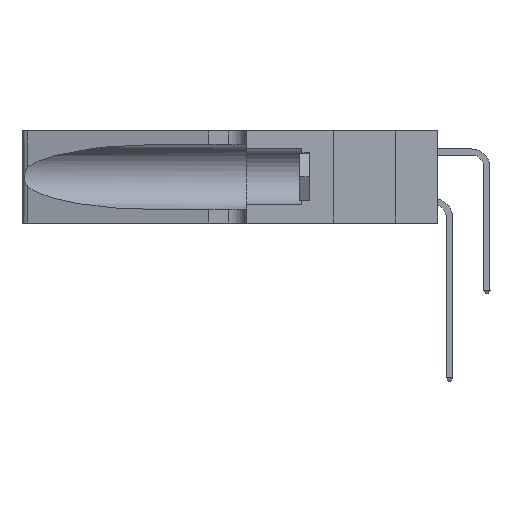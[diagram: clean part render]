
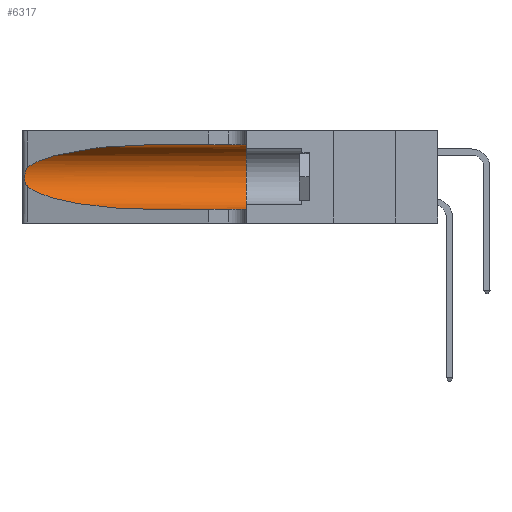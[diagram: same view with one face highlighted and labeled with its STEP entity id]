
A CAD part, left-side view. The second image highlights one B-rep face of the part: STEP entity #6317.
In plain terms, the highlighted cylindrical face has radius 3.308 mm (diameter 6.617 mm), a partial arc.
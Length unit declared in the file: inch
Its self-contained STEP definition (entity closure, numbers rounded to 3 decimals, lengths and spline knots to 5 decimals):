
#1253 = B_SPLINE_CURVE_WITH_KNOTS ( 'NONE', 3,
 ( #28979, #22454, #2146, #24443, #17935, #11226, #15744, #15454, #1946, #20018, #22271, #10839, #24629, #8746 ),
 .UNSPECIFIED., .F., .F.,
 ( 4, 2, 2, 2, 2, 2, 4 ),
 ( 0., 0.00027, 0.00053, 0.00107, 0.0016, 0.00187, 0.00214 ),
 .UNSPECIFIED. ) ;
#1281 = VERTEX_POINT ( 'NONE', #25976 ) ;
#1346 = DIRECTION ( 'NONE',  ( 0., 0., -1. ) ) ;
#1757 = ORIENTED_EDGE ( 'NONE', *, *, #25293, .F. ) ;
#1946 = CARTESIAN_POINT ( 'NONE',  ( 0.26017, 1.23833, 0.17102 ) ) ;
#2146 = CARTESIAN_POINT ( 'NONE',  ( 0.25639, 1.23184, 0.21858 ) ) ;
#2179 = LINE ( 'NONE', #17535, #21235 ) ;
#2608 = CARTESIAN_POINT ( 'NONE',  ( 0.1305, 0.35, 0.05475 ) ) ;
#3270 = CARTESIAN_POINT ( 'NONE',  ( 0.25487, 1.22718, 0.14631 ) ) ;
#3363 = CARTESIAN_POINT ( 'NONE',  ( 0.18966, 0.96281, 0.05475 ) ) ;
#3706 = DIRECTION ( 'NONE',  ( 0., 1., 0. ) ) ;
#3921 = EDGE_CURVE ( 'NONE', #7736, #27381, #5367, .T. ) ;
#5367 = CIRCLE ( 'NONE', #9388, 0.13025 ) ;
#5779 = ORIENTED_EDGE ( 'NONE', *, *, #3921, .F. ) ;
#5825 = CARTESIAN_POINT ( 'NONE',  ( 0.25487, 1.22718, 0.14631 ) ) ;
#6176 = CARTESIAN_POINT ( 'NONE',  ( 0.1305, 0.72297, 0.05475 ) ) ;
#6177 = VERTEX_POINT ( 'NONE', #21495 ) ;
#6317 = ADVANCED_FACE ( 'NONE', ( #8677 ), #25943, .F. ) ;
#7385 = EDGE_CURVE ( 'NONE', #19669, #13662, #17920, .T. ) ;
#7736 = VERTEX_POINT ( 'NONE', #9904 ) ;
#8544 = DIRECTION ( 'NONE',  ( 0., -1., 0. ) ) ;
#8677 = FACE_OUTER_BOUND ( 'NONE', #14441, .T. ) ;
#8746 = CARTESIAN_POINT ( 'NONE',  ( 0.25487, 1.22718, 0.14631 ) ) ;
#8871 = ORIENTED_EDGE ( 'NONE', *, *, #7385, .T. ) ;
#8961 = CARTESIAN_POINT ( 'NONE',  ( 0.18966, 0.96281, 0.31525 ) ) ;
#9388 = AXIS2_PLACEMENT_3D ( 'NONE', #24037, #3706, #12481 ) ;
#9655 = CARTESIAN_POINT ( 'NONE',  ( 0.25487, 1.22718, 0.22369 ) ) ;
#9904 = CARTESIAN_POINT ( 'NONE',  ( 0.1305, 0.35, 0.31525 ) ) ;
#10839 = CARTESIAN_POINT ( 'NONE',  ( 0.25639, 1.23186, 0.15144 ) ) ;
#11226 = CARTESIAN_POINT ( 'NONE',  ( 0.26018, 1.23835, 0.19895 ) ) ;
#11734 = CARTESIAN_POINT ( 'NONE',  ( 0.2373, 1.15595, 0.28018 ) ) ;
#11742 =( BOUNDED_CURVE ( )  B_SPLINE_CURVE ( 3, ( #20508, #8961, #11734, #9655 ),
 .UNSPECIFIED., .F., .T. ) 
 B_SPLINE_CURVE_WITH_KNOTS ( ( 4, 4 ),
 ( 1.5708, 2.84003 ),
 .UNSPECIFIED. ) 
 CURVE ( )  GEOMETRIC_REPRESENTATION_ITEM ( )  RATIONAL_B_SPLINE_CURVE ( ( 1., 0.87, 0.87, 1. ) ) 
 REPRESENTATION_ITEM ( '' )  );
#12386 = ORIENTED_EDGE ( 'NONE', *, *, #16267, .T. ) ;
#12481 = DIRECTION ( 'NONE',  ( 0., 0., 1. ) ) ;
#12581 = DIRECTION ( 'NONE',  ( 0., -1., 0. ) ) ;
#13662 = VERTEX_POINT ( 'NONE', #6176 ) ;
#14441 = EDGE_LOOP ( 'NONE', ( #26100, #16545, #8871, #12386, #5779, #1757 ) ) ;
#15454 = CARTESIAN_POINT ( 'NONE',  ( 0.26075, 1.23896, 0.178 ) ) ;
#15744 = CARTESIAN_POINT ( 'NONE',  ( 0.26075, 1.23896, 0.19203 ) ) ;
#16267 = EDGE_CURVE ( 'NONE', #13662, #27381, #22218, .T. ) ;
#16545 = ORIENTED_EDGE ( 'NONE', *, *, #25419, .T. ) ;
#16970 = CARTESIAN_POINT ( 'NONE',  ( 0.1305, 0.72297, 0.05475 ) ) ;
#17006 = CARTESIAN_POINT ( 'NONE',  ( 0.1305, 1.61858, 0.185 ) ) ;
#17535 = CARTESIAN_POINT ( 'NONE',  ( 0.1305, 1.61858, 0.31525 ) ) ;
#17920 =( BOUNDED_CURVE ( )  B_SPLINE_CURVE ( 3, ( #5825, #25914, #3363, #16970 ),
 .UNSPECIFIED., .F., .F. ) 
 B_SPLINE_CURVE_WITH_KNOTS ( ( 4, 4 ),
 ( 3.44316, 4.71239 ),
 .UNSPECIFIED. ) 
 CURVE ( )  GEOMETRIC_REPRESENTATION_ITEM ( )  RATIONAL_B_SPLINE_CURVE ( ( 1., 0.87, 0.87, 1. ) ) 
 REPRESENTATION_ITEM ( '' )  );
#17935 = CARTESIAN_POINT ( 'NONE',  ( 0.25854, 1.2359, 0.20912 ) ) ;
#19669 = VERTEX_POINT ( 'NONE', #3270 ) ;
#20018 = CARTESIAN_POINT ( 'NONE',  ( 0.25856, 1.23593, 0.16098 ) ) ;
#20169 = EDGE_CURVE ( 'NONE', #1281, #6177, #11742, .T. ) ;
#20508 = CARTESIAN_POINT ( 'NONE',  ( 0.1305, 0.72297, 0.31525 ) ) ;
#21058 = DIRECTION ( 'NONE',  ( 0., -1., 0. ) ) ;
#21235 = VECTOR ( 'NONE', #8544, 39.37008 ) ;
#21495 = CARTESIAN_POINT ( 'NONE',  ( 0.25487, 1.22718, 0.22369 ) ) ;
#22218 = LINE ( 'NONE', #27903, #23969 ) ;
#22271 = CARTESIAN_POINT ( 'NONE',  ( 0.25789, 1.23486, 0.15765 ) ) ;
#22454 = CARTESIAN_POINT ( 'NONE',  ( 0.25555, 1.22994, 0.2215 ) ) ;
#23969 = VECTOR ( 'NONE', #21058, 39.37008 ) ;
#24037 = CARTESIAN_POINT ( 'NONE',  ( 0.1305, 0.35, 0.185 ) ) ;
#24443 = CARTESIAN_POINT ( 'NONE',  ( 0.25787, 1.23484, 0.2124 ) ) ;
#24629 = CARTESIAN_POINT ( 'NONE',  ( 0.25555, 1.22993, 0.14849 ) ) ;
#25293 = EDGE_CURVE ( 'NONE', #1281, #7736, #2179, .T. ) ;
#25419 = EDGE_CURVE ( 'NONE', #6177, #19669, #1253, .T. ) ;
#25914 = CARTESIAN_POINT ( 'NONE',  ( 0.2373, 1.15595, 0.08982 ) ) ;
#25943 = CYLINDRICAL_SURFACE ( 'NONE', #27389, 0.13025 ) ;
#25976 = CARTESIAN_POINT ( 'NONE',  ( 0.1305, 0.72297, 0.31525 ) ) ;
#26100 = ORIENTED_EDGE ( 'NONE', *, *, #20169, .T. ) ;
#27381 = VERTEX_POINT ( 'NONE', #2608 ) ;
#27389 = AXIS2_PLACEMENT_3D ( 'NONE', #17006, #12581, #1346 ) ;
#27903 = CARTESIAN_POINT ( 'NONE',  ( 0.1305, 1.61858, 0.05475 ) ) ;
#28979 = CARTESIAN_POINT ( 'NONE',  ( 0.25487, 1.22718, 0.22369 ) ) ;
